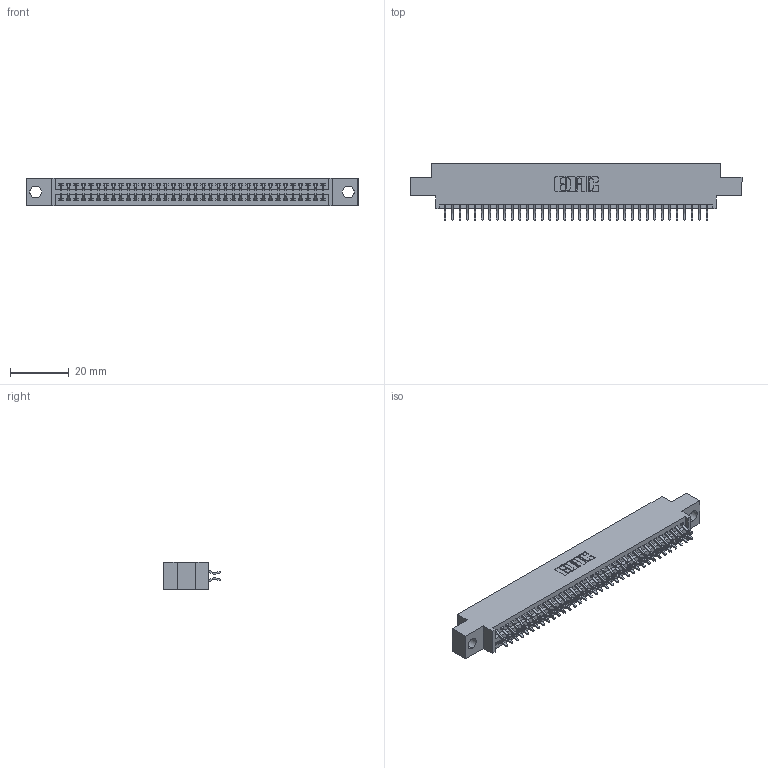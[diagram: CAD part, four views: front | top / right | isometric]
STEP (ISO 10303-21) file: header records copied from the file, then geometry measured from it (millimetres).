
FILE_DESCRIPTION (( 'STEP AP203' ), '1' );
FILE_NAME ('345-072-556-804.STEP', '2021-05-20T09:06:01', ( '' ), ( '' ), 'SwSTEP 2.0', 'SolidWorks 2020', '' );
FILE_SCHEMA (( 'CONFIG_CONTROL_DESIGN' ));
Length unit declared in the file: inch
Products named in the file (3): 345-072-556-804; 345 Part_0.170 Offset - 0.156 Dia-TI; 345-292-001_556 Tail
Assembly tree (73 placements, depth 2):
  345-072-556-804
    345 Part_0.170 Offset - 0.156 Dia-TI
    345-292-001_556 Tail  x72
Bounding box: 112.65 x 19.24 x 9.4 mm (x, y, z)
Volume: 10665 mm3; surface area: 15580.4 mm2
Topology: 73 solids, 73 shells, 4176 faces, 12413 edges, 8178 vertices
Faces by surface type: plane 2762, cylinder 1414
Entity records: 29825 total; most frequent: CARTESIAN_POINT 5026, ORIENTED_EDGE 4946, DIRECTION 4425, EDGE_CURVE 2473, VECTOR 2189, LINE 2189, VERTEX_POINT 1646, AXIS2_PLACEMENT_3D 1118
